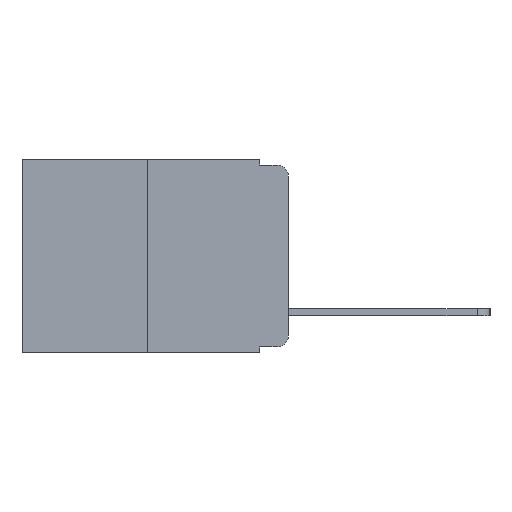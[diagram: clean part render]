
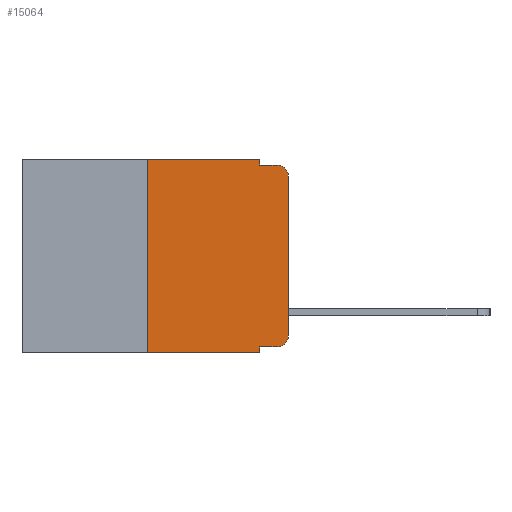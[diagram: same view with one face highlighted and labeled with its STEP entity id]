
A CAD part, left-side view. The second image highlights one B-rep face of the part: STEP entity #15064.
In plain terms, the highlighted planar face has unit normal (-1, 0, 0).
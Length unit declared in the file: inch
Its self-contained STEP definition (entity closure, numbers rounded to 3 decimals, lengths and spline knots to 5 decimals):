
#466 = LINE ( 'NONE', #11836, #14457 ) ;
#857 = DIRECTION ( 'NONE',  ( 0., 0., -1. ) ) ;
#977 = AXIS2_PLACEMENT_3D ( 'NONE', #10629, #10582, #2953 ) ;
#1591 = ORIENTED_EDGE ( 'NONE', *, *, #16022, .T. ) ;
#2398 = CARTESIAN_POINT ( 'NONE',  ( 0., 0., -0.03 ) ) ;
#2953 = DIRECTION ( 'NONE',  ( 0., 0., -1. ) ) ;
#3038 = EDGE_CURVE ( 'NONE', #5037, #7693, #17662, .T. ) ;
#3422 = CARTESIAN_POINT ( 'NONE',  ( 0., 0.051, -0.01 ) ) ;
#3520 = CARTESIAN_POINT ( 'NONE',  ( 0., 0.051, -0.333 ) ) ;
#3599 = EDGE_CURVE ( 'NONE', #17740, #5229, #9363, .T. ) ;
#3693 = LINE ( 'NONE', #15798, #10781 ) ;
#3735 = CARTESIAN_POINT ( 'NONE',  ( 0., 0.051, -0.01 ) ) ;
#3900 = DIRECTION ( 'NONE',  ( 0., -1., 0. ) ) ;
#3941 = CARTESIAN_POINT ( 'NONE',  ( 0., 0.02, -0.313 ) ) ;
#3942 = EDGE_CURVE ( 'NONE', #7693, #15914, #11081, .T. ) ;
#3976 = AXIS2_PLACEMENT_3D ( 'NONE', #7092, #16523, #8533 ) ;
#4410 = LINE ( 'NONE', #6943, #14561 ) ;
#4558 = EDGE_CURVE ( 'NONE', #15914, #17740, #5556, .T. ) ;
#4696 = ORIENTED_EDGE ( 'NONE', *, *, #3942, .T. ) ;
#4736 = DIRECTION ( 'NONE',  ( 0., -1., 0. ) ) ;
#4881 = ORIENTED_EDGE ( 'NONE', *, *, #12373, .F. ) ;
#5019 = LINE ( 'NONE', #8152, #8362 ) ;
#5037 = VERTEX_POINT ( 'NONE', #8211 ) ;
#5159 = CARTESIAN_POINT ( 'NONE',  ( 0., 0.051, 0. ) ) ;
#5170 = VERTEX_POINT ( 'NONE', #13968 ) ;
#5189 = DIRECTION ( 'NONE',  ( 0., -1., 0. ) ) ;
#5229 = VERTEX_POINT ( 'NONE', #7158 ) ;
#5442 = VERTEX_POINT ( 'NONE', #12540 ) ;
#5502 = CARTESIAN_POINT ( 'NONE',  ( 0., 0.051, 0. ) ) ;
#5556 = LINE ( 'NONE', #16266, #15987 ) ;
#5614 = PLANE ( 'NONE',  #3976 ) ;
#5692 = FACE_OUTER_BOUND ( 'NONE', #7346, .T. ) ;
#6055 = VERTEX_POINT ( 'NONE', #12277 ) ;
#6943 = CARTESIAN_POINT ( 'NONE',  ( 0., 0.25, 0. ) ) ;
#7092 = CARTESIAN_POINT ( 'NONE',  ( 0., 0.473, 0. ) ) ;
#7158 = CARTESIAN_POINT ( 'NONE',  ( 0., 0.02, -0.01 ) ) ;
#7308 = DIRECTION ( 'NONE',  ( 0., 0., -1. ) ) ;
#7346 = EDGE_LOOP ( 'NONE', ( #8538, #12332, #4881, #16379, #13219, #15834, #1591, #14657, #17693, #4696 ) ) ;
#7693 = VERTEX_POINT ( 'NONE', #17421 ) ;
#7806 = EDGE_CURVE ( 'NONE', #5442, #5170, #4410, .T. ) ;
#8152 = CARTESIAN_POINT ( 'NONE',  ( 0., 0.473, 0. ) ) ;
#8211 = CARTESIAN_POINT ( 'NONE',  ( 0., 0.051, -0.333 ) ) ;
#8362 = VECTOR ( 'NONE', #3900, 39.37008 ) ;
#8533 = DIRECTION ( 'NONE',  ( 0., 0., -1. ) ) ;
#8538 = ORIENTED_EDGE ( 'NONE', *, *, #4558, .T. ) ;
#8742 = EDGE_CURVE ( 'NONE', #5037, #6055, #3693, .T. ) ;
#8913 = CARTESIAN_POINT ( 'NONE',  ( 0., 0., -0.313 ) ) ;
#9363 = CIRCLE ( 'NONE', #977, 0.02 ) ;
#10425 = LINE ( 'NONE', #5159, #17433 ) ;
#10582 = DIRECTION ( 'NONE',  ( -1., 0., 0. ) ) ;
#10629 = CARTESIAN_POINT ( 'NONE',  ( 0., 0.02, -0.03 ) ) ;
#10781 = VECTOR ( 'NONE', #17112, 39.37008 ) ;
#11081 = CIRCLE ( 'NONE', #16673, 0.02 ) ;
#11085 = LINE ( 'NONE', #3735, #13769 ) ;
#11104 = VECTOR ( 'NONE', #4736, 39.37008 ) ;
#11111 = VERTEX_POINT ( 'NONE', #5502 ) ;
#11836 = CARTESIAN_POINT ( 'NONE',  ( 0., 0.473, -0.343 ) ) ;
#12277 = CARTESIAN_POINT ( 'NONE',  ( 0., 0.051, -0.343 ) ) ;
#12332 = ORIENTED_EDGE ( 'NONE', *, *, #3599, .T. ) ;
#12373 = EDGE_CURVE ( 'NONE', #15320, #5229, #11085, .T. ) ;
#12540 = CARTESIAN_POINT ( 'NONE',  ( 0., 0.25, -0.343 ) ) ;
#13190 = DIRECTION ( 'NONE',  ( 0., -1., 0. ) ) ;
#13219 = ORIENTED_EDGE ( 'NONE', *, *, #14940, .F. ) ;
#13294 = EDGE_CURVE ( 'NONE', #11111, #15320, #10425, .T. ) ;
#13769 = VECTOR ( 'NONE', #5189, 39.37008 ) ;
#13968 = CARTESIAN_POINT ( 'NONE',  ( 0., 0.25, 0. ) ) ;
#14314 = DIRECTION ( 'NONE',  ( -1., 0., 0. ) ) ;
#14457 = VECTOR ( 'NONE', #13190, 39.37008 ) ;
#14561 = VECTOR ( 'NONE', #15089, 39.37008 ) ;
#14657 = ORIENTED_EDGE ( 'NONE', *, *, #8742, .F. ) ;
#14940 = EDGE_CURVE ( 'NONE', #5170, #11111, #5019, .T. ) ;
#15064 = ADVANCED_FACE ( 'NONE', ( #5692 ), #5614, .F. ) ;
#15089 = DIRECTION ( 'NONE',  ( 0., 0., 1. ) ) ;
#15320 = VERTEX_POINT ( 'NONE', #3422 ) ;
#15798 = CARTESIAN_POINT ( 'NONE',  ( 0., 0.051, 0. ) ) ;
#15834 = ORIENTED_EDGE ( 'NONE', *, *, #7806, .F. ) ;
#15914 = VERTEX_POINT ( 'NONE', #8913 ) ;
#15987 = VECTOR ( 'NONE', #16286, 39.37008 ) ;
#16022 = EDGE_CURVE ( 'NONE', #5442, #6055, #466, .T. ) ;
#16266 = CARTESIAN_POINT ( 'NONE',  ( 0., 0., 0. ) ) ;
#16286 = DIRECTION ( 'NONE',  ( 0., 0., 1. ) ) ;
#16379 = ORIENTED_EDGE ( 'NONE', *, *, #13294, .F. ) ;
#16523 = DIRECTION ( 'NONE',  ( 1., 0., 0. ) ) ;
#16673 = AXIS2_PLACEMENT_3D ( 'NONE', #3941, #14314, #7308 ) ;
#17112 = DIRECTION ( 'NONE',  ( 0., 0., -1. ) ) ;
#17421 = CARTESIAN_POINT ( 'NONE',  ( 0., 0.02, -0.333 ) ) ;
#17433 = VECTOR ( 'NONE', #857, 39.37008 ) ;
#17662 = LINE ( 'NONE', #3520, #11104 ) ;
#17693 = ORIENTED_EDGE ( 'NONE', *, *, #3038, .T. ) ;
#17740 = VERTEX_POINT ( 'NONE', #2398 ) ;
